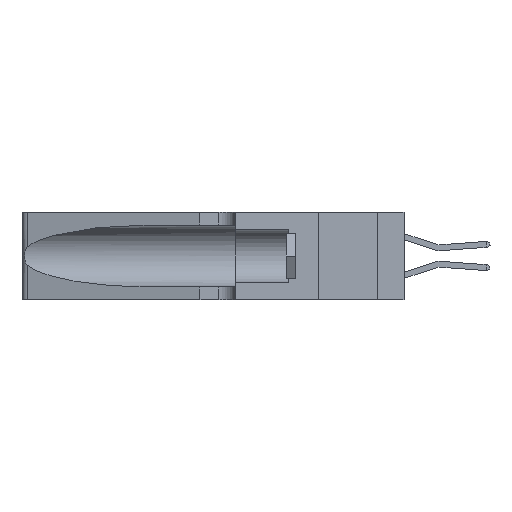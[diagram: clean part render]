
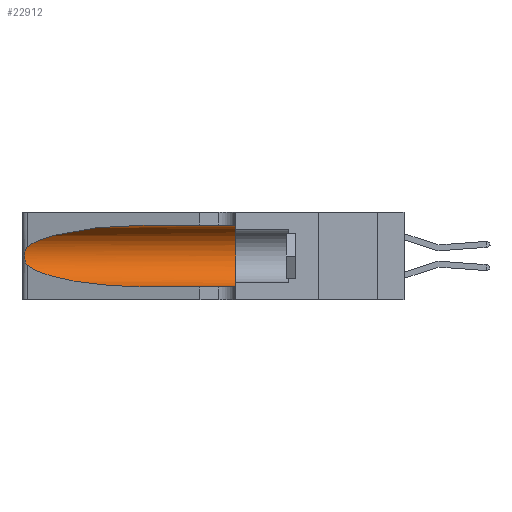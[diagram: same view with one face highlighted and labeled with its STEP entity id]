
A CAD part, left-side view. The second image highlights one B-rep face of the part: STEP entity #22912.
In plain terms, the highlighted cylindrical face has radius 3.308 mm (diameter 6.617 mm), a partial arc.
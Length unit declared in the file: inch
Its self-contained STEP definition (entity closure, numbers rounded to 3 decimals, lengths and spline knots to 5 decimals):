
#427 = VECTOR ( 'NONE', #7379, 39.37008 ) ;
#2018 = LINE ( 'NONE', #9297, #16161 ) ;
#3392 = DIRECTION ( 'NONE',  ( 0., 1., 0. ) ) ;
#3686 = CARTESIAN_POINT ( 'NONE',  ( 0.26017, 1.23833, 0.17102 ) ) ;
#3992 = VERTEX_POINT ( 'NONE', #23636 ) ;
#4804 = EDGE_CURVE ( 'NONE', #34490, #3992, #32335, .T. ) ;
#4831 = CARTESIAN_POINT ( 'NONE',  ( 0.1305, 0.35, 0.31525 ) ) ;
#4991 = CARTESIAN_POINT ( 'NONE',  ( 0.1305, 0.72297, 0.31525 ) ) ;
#5010 = CARTESIAN_POINT ( 'NONE',  ( 0.1305, 1.61858, 0.05475 ) ) ;
#5277 = LINE ( 'NONE', #5010, #427 ) ;
#5826 = CARTESIAN_POINT ( 'NONE',  ( 0.1305, 0.35, 0.05475 ) ) ;
#6663 = CARTESIAN_POINT ( 'NONE',  ( 0.25787, 1.23484, 0.2124 ) ) ;
#7027 = CARTESIAN_POINT ( 'NONE',  ( 0.25487, 1.22718, 0.22369 ) ) ;
#7379 = DIRECTION ( 'NONE',  ( 0., -1., 0. ) ) ;
#7985 = EDGE_LOOP ( 'NONE', ( #12053, #24578, #32984, #29741, #14361, #12274 ) ) ;
#8369 = CARTESIAN_POINT ( 'NONE',  ( 0.1305, 0.35, 0.185 ) ) ;
#9286 = VERTEX_POINT ( 'NONE', #4831 ) ;
#9297 = CARTESIAN_POINT ( 'NONE',  ( 0.1305, 1.61858, 0.31525 ) ) ;
#9874 = CARTESIAN_POINT ( 'NONE',  ( 0.25555, 1.22993, 0.14849 ) ) ;
#9983 = EDGE_CURVE ( 'NONE', #33198, #33929, #26822, .T. ) ;
#10654 = CARTESIAN_POINT ( 'NONE',  ( 0.2373, 1.15595, 0.28018 ) ) ;
#10782 = DIRECTION ( 'NONE',  ( 0., 0., -1. ) ) ;
#12053 = ORIENTED_EDGE ( 'NONE', *, *, #4804, .T. ) ;
#12274 = ORIENTED_EDGE ( 'NONE', *, *, #35231, .F. ) ;
#12580 = CARTESIAN_POINT ( 'NONE',  ( 0.25487, 1.22718, 0.14631 ) ) ;
#13491 = CARTESIAN_POINT ( 'NONE',  ( 0.18966, 0.96281, 0.05475 ) ) ;
#14361 = ORIENTED_EDGE ( 'NONE', *, *, #17311, .F. ) ;
#15291 = CARTESIAN_POINT ( 'NONE',  ( 0.25639, 1.23186, 0.15144 ) ) ;
#15414 = CARTESIAN_POINT ( 'NONE',  ( 0.25789, 1.23486, 0.15765 ) ) ;
#15539 = CARTESIAN_POINT ( 'NONE',  ( 0.25854, 1.2359, 0.20912 ) ) ;
#16079 = CARTESIAN_POINT ( 'NONE',  ( 0.1305, 1.61858, 0.185 ) ) ;
#16161 = VECTOR ( 'NONE', #23119, 39.37008 ) ;
#16321 = CARTESIAN_POINT ( 'NONE',  ( 0.25487, 1.22718, 0.22369 ) ) ;
#17311 = EDGE_CURVE ( 'NONE', #9286, #26980, #19212, .T. ) ;
#17844 = AXIS2_PLACEMENT_3D ( 'NONE', #16079, #24750, #10782 ) ;
#17969 = CARTESIAN_POINT ( 'NONE',  ( 0.25555, 1.22994, 0.2215 ) ) ;
#18729 = AXIS2_PLACEMENT_3D ( 'NONE', #8369, #3392, #20198 ) ;
#19212 = CIRCLE ( 'NONE', #18729, 0.13025 ) ;
#19402 = CARTESIAN_POINT ( 'NONE',  ( 0.1305, 0.72297, 0.05475 ) ) ;
#20198 = DIRECTION ( 'NONE',  ( 0., 0., 1. ) ) ;
#21112 = CARTESIAN_POINT ( 'NONE',  ( 0.26075, 1.23896, 0.19203 ) ) ;
#21650 = CARTESIAN_POINT ( 'NONE',  ( 0.25487, 1.22718, 0.14631 ) ) ;
#22912 = ADVANCED_FACE ( 'NONE', ( #28917 ), #24043, .F. ) ;
#23119 = DIRECTION ( 'NONE',  ( 0., -1., 0. ) ) ;
#23636 = CARTESIAN_POINT ( 'NONE',  ( 0.25487, 1.22718, 0.22369 ) ) ;
#23721 = CARTESIAN_POINT ( 'NONE',  ( 0.25639, 1.23184, 0.21858 ) ) ;
#24043 = CYLINDRICAL_SURFACE ( 'NONE', #17844, 0.13025 ) ;
#24578 = ORIENTED_EDGE ( 'NONE', *, *, #32417, .T. ) ;
#24750 = DIRECTION ( 'NONE',  ( 0., -1., 0. ) ) ;
#24838 = CARTESIAN_POINT ( 'NONE',  ( 0.25487, 1.22718, 0.14631 ) ) ;
#25261 = CARTESIAN_POINT ( 'NONE',  ( 0.1305, 0.72297, 0.31525 ) ) ;
#26436 = CARTESIAN_POINT ( 'NONE',  ( 0.26018, 1.23835, 0.19895 ) ) ;
#26822 =( BOUNDED_CURVE ( )  B_SPLINE_CURVE ( 3, ( #21650, #27484, #13491, #19402 ),
 .UNSPECIFIED., .F., .T. ) 
 B_SPLINE_CURVE_WITH_KNOTS ( ( 4, 4 ),
 ( 3.44316, 4.71239 ),
 .UNSPECIFIED. ) 
 CURVE ( )  GEOMETRIC_REPRESENTATION_ITEM ( )  RATIONAL_B_SPLINE_CURVE ( ( 1., 0.87, 0.87, 1. ) ) 
 REPRESENTATION_ITEM ( '' )  );
#26980 = VERTEX_POINT ( 'NONE', #5826 ) ;
#27484 = CARTESIAN_POINT ( 'NONE',  ( 0.2373, 1.15595, 0.08982 ) ) ;
#28381 = B_SPLINE_CURVE_WITH_KNOTS ( 'NONE', 3,
 ( #7027, #17969, #23721, #6663, #15539, #26436, #21112, #32567, #3686, #29319, #15414, #15291, #9874, #12580 ),
 .UNSPECIFIED., .F., .F.,
 ( 4, 2, 2, 2, 2, 2, 4 ),
 ( 0., 0.00027, 0.00053, 0.00107, 0.0016, 0.00187, 0.00214 ),
 .UNSPECIFIED. ) ;
#28917 = FACE_OUTER_BOUND ( 'NONE', #7985, .T. ) ;
#29319 = CARTESIAN_POINT ( 'NONE',  ( 0.25856, 1.23593, 0.16098 ) ) ;
#29741 = ORIENTED_EDGE ( 'NONE', *, *, #30742, .T. ) ;
#30742 = EDGE_CURVE ( 'NONE', #33929, #26980, #5277, .T. ) ;
#32335 =( BOUNDED_CURVE ( )  B_SPLINE_CURVE ( 3, ( #25261, #33485, #10654, #16321 ),
 .UNSPECIFIED., .F., .F. ) 
 B_SPLINE_CURVE_WITH_KNOTS ( ( 4, 4 ),
 ( 1.5708, 2.84003 ),
 .UNSPECIFIED. ) 
 CURVE ( )  GEOMETRIC_REPRESENTATION_ITEM ( )  RATIONAL_B_SPLINE_CURVE ( ( 1., 0.87, 0.87, 1. ) ) 
 REPRESENTATION_ITEM ( '' )  );
#32417 = EDGE_CURVE ( 'NONE', #3992, #33198, #28381, .T. ) ;
#32567 = CARTESIAN_POINT ( 'NONE',  ( 0.26075, 1.23896, 0.178 ) ) ;
#32984 = ORIENTED_EDGE ( 'NONE', *, *, #9983, .T. ) ;
#33198 = VERTEX_POINT ( 'NONE', #24838 ) ;
#33485 = CARTESIAN_POINT ( 'NONE',  ( 0.18966, 0.96281, 0.31525 ) ) ;
#33929 = VERTEX_POINT ( 'NONE', #34053 ) ;
#34053 = CARTESIAN_POINT ( 'NONE',  ( 0.1305, 0.72297, 0.05475 ) ) ;
#34490 = VERTEX_POINT ( 'NONE', #4991 ) ;
#35231 = EDGE_CURVE ( 'NONE', #34490, #9286, #2018, .T. ) ;
